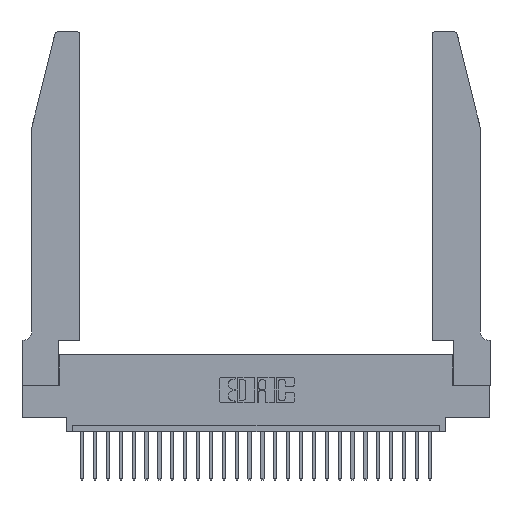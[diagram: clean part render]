
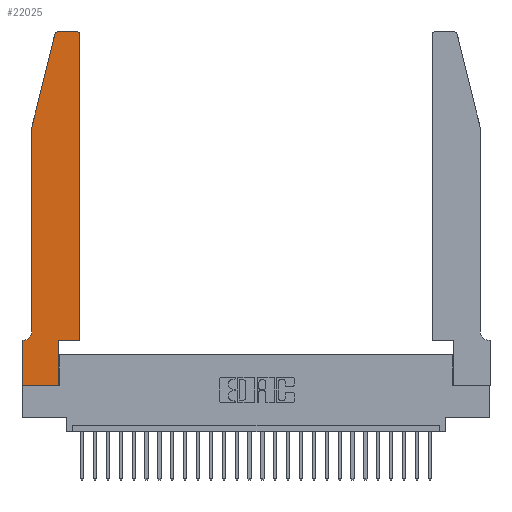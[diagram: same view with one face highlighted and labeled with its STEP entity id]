
A CAD part, top view. The second image highlights one B-rep face of the part: STEP entity #22025.
In plain terms, the highlighted planar face has unit normal (0, 0, 1).
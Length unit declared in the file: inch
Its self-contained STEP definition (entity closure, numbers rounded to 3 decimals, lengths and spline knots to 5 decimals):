
#58 = DIRECTION ( 'NONE',  ( 0., 1., 0. ) ) ;
#408 = VERTEX_POINT ( 'NONE', #3255 ) ;
#625 = CARTESIAN_POINT ( 'NONE',  ( 0., 0., 0.37 ) ) ;
#1186 = VERTEX_POINT ( 'NONE', #625 ) ;
#1361 = VECTOR ( 'NONE', #2100, 39.37008 ) ;
#1393 = DIRECTION ( 'NONE',  ( 1., 0., 0. ) ) ;
#1657 = CARTESIAN_POINT ( 'NONE',  ( 0., 0.35, 0.37 ) ) ;
#1673 = EDGE_CURVE ( 'NONE', #1186, #16587, #26271, .T. ) ;
#1975 = LINE ( 'NONE', #13214, #12052 ) ;
#1983 = LINE ( 'NONE', #19420, #14767 ) ;
#2100 = DIRECTION ( 'NONE',  ( 1., 0., 0. ) ) ;
#2249 = AXIS2_PLACEMENT_3D ( 'NONE', #17814, #21942, #19958 ) ;
#2413 = CARTESIAN_POINT ( 'NONE',  ( 0.4505, 2.72, 0.37 ) ) ;
#3250 = EDGE_CURVE ( 'NONE', #14170, #14457, #1975, .T. ) ;
#3255 = CARTESIAN_POINT ( 'NONE',  ( 0.284, 2.75, 0.37 ) ) ;
#3779 = EDGE_CURVE ( 'NONE', #408, #24039, #20072, .T. ) ;
#3830 = CARTESIAN_POINT ( 'NONE',  ( 0.4205, 2.72, 0.37 ) ) ;
#4247 = CARTESIAN_POINT ( 'NONE',  ( 0., 0., 0.37 ) ) ;
#4260 = CARTESIAN_POINT ( 'NONE',  ( 0.25487, 2.72718, 0.37 ) ) ;
#4311 = DIRECTION ( 'NONE',  ( 1., 0., 0. ) ) ;
#4615 = DIRECTION ( 'NONE',  ( -1., 0., 0. ) ) ;
#4662 = VECTOR ( 'NONE', #26287, 39.37008 ) ;
#5299 = EDGE_CURVE ( 'NONE', #24039, #26181, #15802, .T. ) ;
#5999 = DIRECTION ( 'NONE',  ( 0., 0., 1. ) ) ;
#6402 = CARTESIAN_POINT ( 'NONE',  ( 0.0755, 2., 0.37 ) ) ;
#6923 = ORIENTED_EDGE ( 'NONE', *, *, #18418, .T. ) ;
#7441 = LINE ( 'NONE', #23842, #25587 ) ;
#8072 = CARTESIAN_POINT ( 'NONE',  ( 0.4505, 0.35, 0.37 ) ) ;
#8370 = CARTESIAN_POINT ( 'NONE',  ( 0.4505, 0.35, 0.37 ) ) ;
#8651 = DIRECTION ( 'NONE',  ( -0.239, -0.971, 0. ) ) ;
#8736 = AXIS2_PLACEMENT_3D ( 'NONE', #3830, #5999, #22859 ) ;
#9207 = ORIENTED_EDGE ( 'NONE', *, *, #16102, .T. ) ;
#9268 = VERTEX_POINT ( 'NONE', #15526 ) ;
#9404 = CARTESIAN_POINT ( 'NONE',  ( 0.0755, 2., 0.37 ) ) ;
#10117 = CARTESIAN_POINT ( 'NONE',  ( 0.2865, 0.35, 0.37 ) ) ;
#10365 = ORIENTED_EDGE ( 'NONE', *, *, #26682, .T. ) ;
#10427 = EDGE_CURVE ( 'NONE', #23284, #1186, #18836, .T. ) ;
#10964 = VERTEX_POINT ( 'NONE', #10117 ) ;
#11246 = CARTESIAN_POINT ( 'NONE',  ( 0.2605, 2.75, 0.37 ) ) ;
#11903 = ORIENTED_EDGE ( 'NONE', *, *, #18334, .T. ) ;
#12052 = VECTOR ( 'NONE', #17534, 39.37008 ) ;
#12694 = AXIS2_PLACEMENT_3D ( 'NONE', #17190, #21674, #4311 ) ;
#13067 = CARTESIAN_POINT ( 'NONE',  ( 0.0755, 0.35, 0.37 ) ) ;
#13153 = VECTOR ( 'NONE', #20925, 39.37008 ) ;
#13214 = CARTESIAN_POINT ( 'NONE',  ( 0.4505, 0.35, 0.37 ) ) ;
#14170 = VERTEX_POINT ( 'NONE', #8370 ) ;
#14457 = VERTEX_POINT ( 'NONE', #2413 ) ;
#14767 = VECTOR ( 'NONE', #20998, 39.37008 ) ;
#14829 = LINE ( 'NONE', #13067, #25581 ) ;
#15107 = VECTOR ( 'NONE', #8651, 39.37008 ) ;
#15134 = CARTESIAN_POINT ( 'NONE',  ( 0., 0., 0.37 ) ) ;
#15402 = CARTESIAN_POINT ( 'NONE',  ( 0.2865, 0., 0.37 ) ) ;
#15526 = CARTESIAN_POINT ( 'NONE',  ( 0.4205, 2.75, 0.37 ) ) ;
#15571 = ORIENTED_EDGE ( 'NONE', *, *, #22965, .T. ) ;
#15802 = LINE ( 'NONE', #6402, #15107 ) ;
#16056 = EDGE_CURVE ( 'NONE', #10964, #14170, #25184, .T. ) ;
#16102 = EDGE_CURVE ( 'NONE', #14457, #9268, #24518, .T. ) ;
#16587 = VERTEX_POINT ( 'NONE', #15402 ) ;
#16956 = ORIENTED_EDGE ( 'NONE', *, *, #3779, .T. ) ;
#17190 = CARTESIAN_POINT ( 'NONE',  ( 0.284, 2.72, 0.37 ) ) ;
#17534 = DIRECTION ( 'NONE',  ( 0., 1., 0. ) ) ;
#17814 = CARTESIAN_POINT ( 'NONE',  ( 0., 0.35, 0.37 ) ) ;
#18334 = EDGE_CURVE ( 'NONE', #26181, #23418, #1983, .T. ) ;
#18418 = EDGE_CURVE ( 'NONE', #9268, #408, #18763, .T. ) ;
#18738 = CIRCLE ( 'NONE', #22841, 0.07 ) ;
#18763 = LINE ( 'NONE', #11246, #4662 ) ;
#18836 = LINE ( 'NONE', #15134, #13153 ) ;
#18927 = ORIENTED_EDGE ( 'NONE', *, *, #16056, .T. ) ;
#19420 = CARTESIAN_POINT ( 'NONE',  ( 0.0755, 2., 0.37 ) ) ;
#19453 = VECTOR ( 'NONE', #1393, 39.37008 ) ;
#19704 = CARTESIAN_POINT ( 'NONE',  ( 0.0055, 0.42, 0.37 ) ) ;
#19958 = DIRECTION ( 'NONE',  ( 1., 0., 0. ) ) ;
#20072 = CIRCLE ( 'NONE', #12694, 0.03 ) ;
#20925 = DIRECTION ( 'NONE',  ( 0., -1., 0. ) ) ;
#20998 = DIRECTION ( 'NONE',  ( 0., -1., 0. ) ) ;
#21294 = CARTESIAN_POINT ( 'NONE',  ( 0.0755, 0.42, 0.37 ) ) ;
#21674 = DIRECTION ( 'NONE',  ( 0., 0., 1. ) ) ;
#21942 = DIRECTION ( 'NONE',  ( 0., 0., 1. ) ) ;
#22025 = ADVANCED_FACE ( 'NONE', ( #23988 ), #26556, .T. ) ;
#22841 = AXIS2_PLACEMENT_3D ( 'NONE', #19704, #24136, #24049 ) ;
#22859 = DIRECTION ( 'NONE',  ( 1., 0., 0. ) ) ;
#22965 = EDGE_CURVE ( 'NONE', #23744, #23284, #14829, .T. ) ;
#23284 = VERTEX_POINT ( 'NONE', #1657 ) ;
#23418 = VERTEX_POINT ( 'NONE', #21294 ) ;
#23505 = EDGE_CURVE ( 'NONE', #16587, #10964, #7441, .T. ) ;
#23744 = VERTEX_POINT ( 'NONE', #26079 ) ;
#23842 = CARTESIAN_POINT ( 'NONE',  ( 0.2865, 0.35, 0.37 ) ) ;
#23988 = FACE_OUTER_BOUND ( 'NONE', #25476, .T. ) ;
#24039 = VERTEX_POINT ( 'NONE', #4260 ) ;
#24049 = DIRECTION ( 'NONE',  ( -1., 0., 0. ) ) ;
#24136 = DIRECTION ( 'NONE',  ( 0., 0., -1. ) ) ;
#24510 = ORIENTED_EDGE ( 'NONE', *, *, #23505, .T. ) ;
#24518 = CIRCLE ( 'NONE', #8736, 0.03 ) ;
#24551 = ORIENTED_EDGE ( 'NONE', *, *, #5299, .T. ) ;
#25142 = ORIENTED_EDGE ( 'NONE', *, *, #10427, .T. ) ;
#25184 = LINE ( 'NONE', #8072, #19453 ) ;
#25476 = EDGE_LOOP ( 'NONE', ( #6923, #16956, #24551, #11903, #10365, #15571, #25142, #27578, #24510, #18927, #26844, #9207 ) ) ;
#25581 = VECTOR ( 'NONE', #4615, 39.37008 ) ;
#25587 = VECTOR ( 'NONE', #58, 39.37008 ) ;
#26079 = CARTESIAN_POINT ( 'NONE',  ( 0.0055, 0.35, 0.37 ) ) ;
#26181 = VERTEX_POINT ( 'NONE', #9404 ) ;
#26271 = LINE ( 'NONE', #4247, #1361 ) ;
#26287 = DIRECTION ( 'NONE',  ( -1., 0., 0. ) ) ;
#26556 = PLANE ( 'NONE',  #2249 ) ;
#26682 = EDGE_CURVE ( 'NONE', #23418, #23744, #18738, .T. ) ;
#26844 = ORIENTED_EDGE ( 'NONE', *, *, #3250, .T. ) ;
#27578 = ORIENTED_EDGE ( 'NONE', *, *, #1673, .T. ) ;
